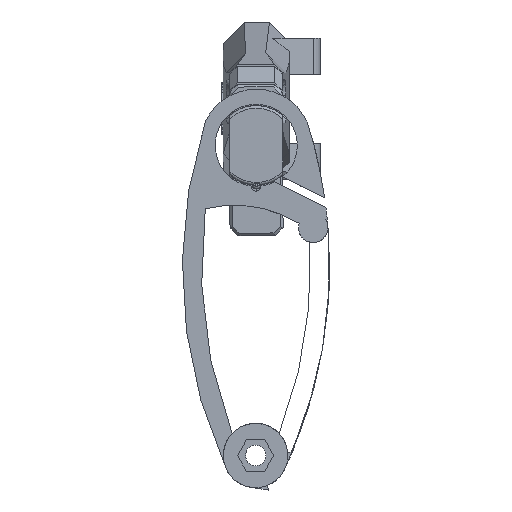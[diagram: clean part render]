
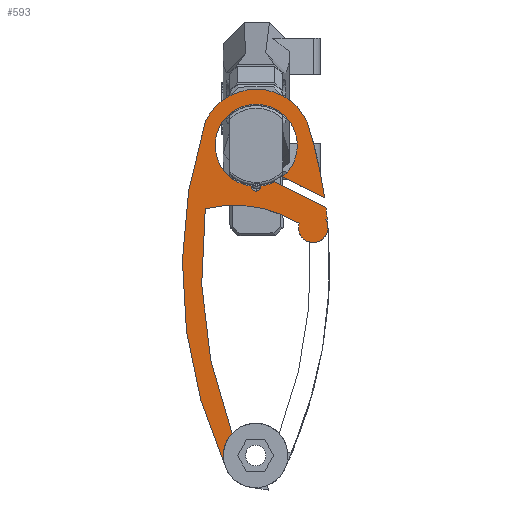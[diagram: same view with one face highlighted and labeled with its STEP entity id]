
A CAD part, front view. The second image highlights one B-rep face of the part: STEP entity #593.
In plain terms, the highlighted planar face has unit normal (0, -1, 0).
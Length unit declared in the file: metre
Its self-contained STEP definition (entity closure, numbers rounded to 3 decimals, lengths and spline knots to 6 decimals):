
#593=ADVANCED_FACE('16:15',(#1379),#1380,.F.);
#1379=FACE_OUTER_BOUND('',#2241,.T.);
#1380=PLANE('',#2242);
#2241=EDGE_LOOP('',(#5285,#5286,#5287,#5288,#5289,#5290,#5291,#5292,#5293,#5294,#5295,#5296,#5297,#5298,#5299,#5300,#5301,#5302,#5303));
#2242=AXIS2_PLACEMENT_3D('',#5304,#5305,#5306);
#5285=ORIENTED_EDGE('',*,*,#6791,.T.);
#5286=ORIENTED_EDGE('',*,*,#6795,.T.);
#5287=ORIENTED_EDGE('',*,*,#6784,.T.);
#5288=ORIENTED_EDGE('',*,*,#6781,.T.);
#5289=ORIENTED_EDGE('',*,*,#6793,.T.);
#5290=ORIENTED_EDGE('',*,*,#6788,.T.);
#5291=ORIENTED_EDGE('',*,*,#6801,.T.);
#5292=ORIENTED_EDGE('',*,*,#6802,.F.);
#5293=ORIENTED_EDGE('',*,*,#6803,.T.);
#5294=ORIENTED_EDGE('',*,*,#6804,.T.);
#5295=ORIENTED_EDGE('',*,*,#6805,.T.);
#5296=ORIENTED_EDGE('',*,*,#6745,.T.);
#5297=ORIENTED_EDGE('',*,*,#6806,.T.);
#5298=ORIENTED_EDGE('',*,*,#6807,.T.);
#5299=ORIENTED_EDGE('',*,*,#6808,.T.);
#5300=ORIENTED_EDGE('',*,*,#6773,.T.);
#5301=ORIENTED_EDGE('',*,*,#6809,.T.);
#5302=ORIENTED_EDGE('',*,*,#6810,.F.);
#5303=ORIENTED_EDGE('',*,*,#6798,.T.);
#5304=CARTESIAN_POINT('',(-0.01739,-0.0005,0.027272));
#5305=DIRECTION('',(0.0,1.0,0.0));
#5306=DIRECTION('',(-1.0,0.0,0.0));
#6745=EDGE_CURVE('16:214',#8422,#8425,#8427,.T.);
#6773=EDGE_CURVE('16:223',#8468,#8480,#8482,.T.);
#6781=EDGE_CURVE('16:187',#8491,#8496,#8498,.F.);
#6784=EDGE_CURVE('16:187',#8500,#8491,#8503,.F.);
#6788=EDGE_CURVE('16:179',#8505,#8509,#8511,.F.);
#6791=EDGE_CURVE('16:167',#8517,#8515,#8518,.F.);
#6793=EDGE_CURVE('16:179',#8496,#8505,#8520,.F.);
#6795=EDGE_CURVE('16:187',#8515,#8500,#8522,.F.);
#6798=EDGE_CURVE('16:193',#8525,#8517,#8526,.T.);
#6801=EDGE_CURVE('16:202',#8509,#8530,#8531,.T.);
#6802=EDGE_CURVE('16:205',#8532,#8530,#8533,.T.);
#6803=EDGE_CURVE('16:208',#8532,#8534,#8535,.T.);
#6804=EDGE_CURVE('16:211',#8534,#8536,#8537,.T.);
#6805=EDGE_CURVE('16:214',#8536,#8422,#8538,.T.);
#6806=EDGE_CURVE('16:217',#8425,#8539,#8540,.T.);
#6807=EDGE_CURVE('16:220',#8539,#8541,#8542,.T.);
#6808=EDGE_CURVE('16:223',#8541,#8468,#8543,.T.);
#6809=EDGE_CURVE('16:226',#8480,#8544,#8545,.T.);
#6810=EDGE_CURVE('16:229',#8525,#8544,#8546,.T.);
#8422=VERTEX_POINT('',#11635);
#8425=VERTEX_POINT('',#11639);
#8427=CIRCLE('',#11642,0.01215);
#8468=VERTEX_POINT('',#11753);
#8480=VERTEX_POINT('',#11768);
#8482=CIRCLE('',#11771,0.005574);
#8491=VERTEX_POINT('',#11782);
#8496=VERTEX_POINT('',#11788);
#8498=CIRCLE('',#11791,0.00175);
#8500=VERTEX_POINT('',#11793);
#8503=CIRCLE('',#11797,0.00175);
#8505=VERTEX_POINT('',#11799);
#8509=VERTEX_POINT('',#11804);
#8511=CIRCLE('',#11807,0.0155);
#8515=VERTEX_POINT('',#11811);
#8517=VERTEX_POINT('',#11814);
#8518=CIRCLE('',#11815,0.0155);
#8520=CIRCLE('',#11818,0.0155);
#8522=CIRCLE('',#11820,0.00175);
#8525=VERTEX_POINT('',#11823);
#8526=LINE('',#11824,#11825);
#8530=VERTEX_POINT('',#11831);
#8531=LINE('',#11832,#11833);
#8532=VERTEX_POINT('',#11834);
#8533=CIRCLE('',#11835,0.180483);
#8534=VERTEX_POINT('',#11836);
#8535=CIRCLE('',#11837,0.02115);
#8536=VERTEX_POINT('',#11838);
#8537=CIRCLE('',#11839,0.180483);
#8538=CIRCLE('',#11840,0.01215);
#8539=VERTEX_POINT('',#11841);
#8540=CIRCLE('',#11842,0.173283);
#8541=VERTEX_POINT('',#11843);
#8542=CIRCLE('',#11844,0.046197);
#8543=CIRCLE('',#11845,0.005574);
#8544=VERTEX_POINT('',#11846);
#8545=LINE('',#11847,#11848);
#8546=CIRCLE('',#11849,0.180483);
#11635=CARTESIAN_POINT('',(-0.005054,-0.0005,0.11973));
#11639=CARTESIAN_POINT('',(-0.008096,-0.0005,0.113818));
#11642=AXIS2_PLACEMENT_3D('',#13568,#13569,#13570);
#11753=CARTESIAN_POINT('',(-0.039345,-0.0005,0.04167));
#11768=CARTESIAN_POINT('',(-0.043175,-0.0005,0.033085));
#11771=AXIS2_PLACEMENT_3D('',#13618,#13619,#13620);
#11782=CARTESIAN_POINT('',(-0.015162,-0.0005,0.02053));
#11788=CARTESIAN_POINT('',(-0.015163,-0.0005,0.020515));
#11791=AXIS2_PLACEMENT_3D('',#13634,#13635,#13636);
#11793=CARTESIAN_POINT('',(-0.018657,-0.0005,0.02071));
#11797=AXIS2_PLACEMENT_3D('',#13641,#13642,#13643);
#11799=CARTESIAN_POINT('',(-0.007999,-0.0005,-0.007522));
#11804=CARTESIAN_POINT('',(-0.02689,-0.0005,0.017027));
#11807=AXIS2_PLACEMENT_3D('',#13649,#13650,#13651);
#11811=CARTESIAN_POINT('',(-0.018657,-0.0005,0.020528));
#11814=CARTESIAN_POINT('',(-0.023985,-0.0005,0.01894));
#11815=AXIS2_PLACEMENT_3D('',#13656,#13657,#13658);
#11818=AXIS2_PLACEMENT_3D('',#13660,#13661,#13662);
#11820=AXIS2_PLACEMENT_3D('',#13666,#13667,#13668);
#11823=CARTESIAN_POINT('',(-0.043308,-0.0005,0.028458));
#11824=CARTESIAN_POINT('',(-0.022085,-0.0005,0.018005));
#11825=VECTOR('',#13675,0.009);
#11831=CARTESIAN_POINT('',(-0.042816,-0.0005,0.024872));
#11832=CARTESIAN_POINT('',(-0.03397,-0.0005,0.020515));
#11833=VECTOR('',#13678,0.009);
#11834=CARTESIAN_POINT('',(-0.036201,-0.0005,-0.003677));
#11835=AXIS2_PLACEMENT_3D('',#13679,#13680,#13681);
#11836=CARTESIAN_POINT('',(0.002267,-0.0005,-0.003677));
#11837=AXIS2_PLACEMENT_3D('',#13682,#13683,#13684);
#11838=CARTESIAN_POINT('',(-0.00558,-0.0005,0.126359));
#11839=AXIS2_PLACEMENT_3D('',#13685,#13686,#13687);
#11840=AXIS2_PLACEMENT_3D('',#13688,#13689,#13690);
#11841=CARTESIAN_POINT('',(0.002198,-0.0005,0.029104));
#11842=AXIS2_PLACEMENT_3D('',#13691,#13692,#13693);
#11843=CARTESIAN_POINT('',(-0.03318,-0.0005,0.034573));
#11844=AXIS2_PLACEMENT_3D('',#13694,#13695,#13696);
#11845=AXIS2_PLACEMENT_3D('',#13697,#13698,#13699);
#11846=CARTESIAN_POINT('',(-0.043793,-0.0005,0.032677));
#11847=CARTESIAN_POINT('',(-0.032436,-0.0005,0.040177));
#11848=VECTOR('',#13700,0.009);
#11849=AXIS2_PLACEMENT_3D('',#13701,#13702,#13703);
#13568=CARTESIAN_POINT('',(-0.016967,-0.0005,0.12212));
#13569=DIRECTION('',(0.0,1.0,0.0));
#13570=DIRECTION('',(-1.0,0.0,0.0));
#13618=CARTESIAN_POINT('',(-0.038524,-0.0005,0.036157));
#13619=DIRECTION('',(0.0,-1.0,0.0));
#13620=DIRECTION('',(-1.0,0.0,0.0));
#13634=CARTESIAN_POINT('',(-0.016909,-0.0005,0.02062));
#13635=DIRECTION('',(-0.0,-1.0,0.0));
#13636=DIRECTION('',(-0.999,0.0,0.051));
#13641=CARTESIAN_POINT('',(-0.016909,-0.0005,0.02062));
#13642=DIRECTION('',(-0.0,-1.0,0.0));
#13643=DIRECTION('',(-0.999,0.0,0.051));
#13649=CARTESIAN_POINT('',(-0.016967,-0.0005,0.00512));
#13650=DIRECTION('',(0.0,-1.0,-0.0));
#13651=DIRECTION('',(0.579,0.0,-0.816));
#13656=CARTESIAN_POINT('',(-0.016967,-0.0005,0.00512));
#13657=DIRECTION('',(0.0,-1.0,-0.0));
#13658=DIRECTION('',(0.091,0.0,-0.996));
#13660=CARTESIAN_POINT('',(-0.016967,-0.0005,0.00512));
#13661=DIRECTION('',(0.0,-1.0,-0.0));
#13662=DIRECTION('',(0.579,0.0,-0.816));
#13666=CARTESIAN_POINT('',(-0.016909,-0.0005,0.02062));
#13667=DIRECTION('',(-0.0,-1.0,0.0));
#13668=DIRECTION('',(-0.999,0.0,0.051));
#13675=DIRECTION('',(0.897,0.0,-0.442));
#13678=DIRECTION('',(-0.897,0.0,0.442));
#13679=CARTESIAN_POINT('',(0.135736,-0.0005,0.051202));
#13680=DIRECTION('',(0.0,1.0,0.0));
#13681=DIRECTION('',(-0.953,0.0,-0.304));
#13682=CARTESIAN_POINT('',(-0.016967,-0.0005,0.00512));
#13683=DIRECTION('',(0.0,-1.0,0.0));
#13684=DIRECTION('',(-1.0,0.0,0.0));
#13685=CARTESIAN_POINT('',(-0.16967,-0.0005,0.051202));
#13686=DIRECTION('',(0.0,-1.0,0.0));
#13687=DIRECTION('',(0.953,0.0,-0.304));
#13688=CARTESIAN_POINT('',(-0.016967,-0.0005,0.12212));
#13689=DIRECTION('',(0.0,1.0,0.0));
#13690=DIRECTION('',(-1.0,0.0,0.0));
#13691=CARTESIAN_POINT('',(-0.16967,-0.0005,0.051202));
#13692=DIRECTION('',(-0.0,1.0,0.0));
#13693=DIRECTION('',(0.908,0.0,0.418));
#13694=CARTESIAN_POINT('',(-0.008985,-0.0005,0.073927));
#13695=DIRECTION('',(0.0,1.0,0.0));
#13696=DIRECTION('',(0.242,0.0,-0.97));
#13697=CARTESIAN_POINT('',(-0.038524,-0.0005,0.036157));
#13698=DIRECTION('',(0.0,-1.0,0.0));
#13699=DIRECTION('',(-1.0,0.0,0.0));
#13700=DIRECTION('',(-0.834,0.0,-0.551));
#13701=CARTESIAN_POINT('',(0.135736,-0.0005,0.051202));
#13702=DIRECTION('',(0.0,1.0,0.0));
#13703=DIRECTION('',(-0.953,0.0,-0.304));
